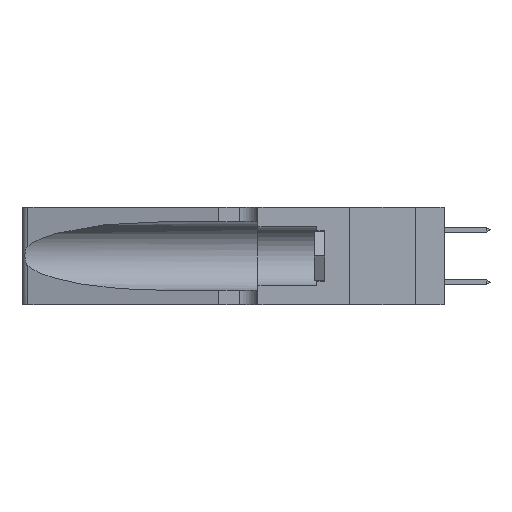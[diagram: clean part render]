
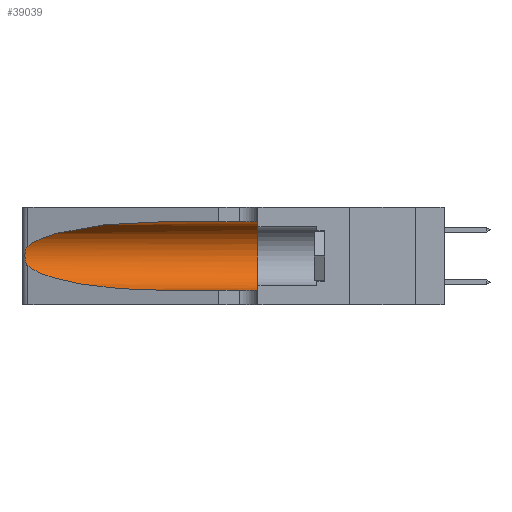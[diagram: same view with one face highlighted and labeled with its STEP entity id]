
A CAD part, left-side view. The second image highlights one B-rep face of the part: STEP entity #39039.
In plain terms, the highlighted cylindrical face has radius 3.308 mm (diameter 6.617 mm), a partial arc.
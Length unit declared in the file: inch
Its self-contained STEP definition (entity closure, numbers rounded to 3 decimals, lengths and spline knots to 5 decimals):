
#1113 = EDGE_CURVE ( 'NONE', #6141, #28850, #5608, .T. ) ;
#3563 =( BOUNDED_CURVE ( )  B_SPLINE_CURVE ( 3, ( #38087, #4190, #41437, #21328 ),
 .UNSPECIFIED., .F., .T. ) 
 B_SPLINE_CURVE_WITH_KNOTS ( ( 4, 4 ),
 ( 3.44316, 4.71239 ),
 .UNSPECIFIED. ) 
 CURVE ( )  GEOMETRIC_REPRESENTATION_ITEM ( )  RATIONAL_B_SPLINE_CURVE ( ( 1., 0.87, 0.87, 1. ) ) 
 REPRESENTATION_ITEM ( '' )  );
#4190 = CARTESIAN_POINT ( 'NONE',  ( 0.2373, 1.15595, 0.08982 ) ) ;
#4416 = CARTESIAN_POINT ( 'NONE',  ( 0.25787, 1.23484, 0.2124 ) ) ;
#5608 = CIRCLE ( 'NONE', #32567, 0.13025 ) ;
#6013 = VERTEX_POINT ( 'NONE', #11095 ) ;
#6141 = VERTEX_POINT ( 'NONE', #38516 ) ;
#6276 = CARTESIAN_POINT ( 'NONE',  ( 0.18966, 0.96281, 0.31525 ) ) ;
#7847 = CARTESIAN_POINT ( 'NONE',  ( 0.26018, 1.23835, 0.19895 ) ) ;
#7897 = ORIENTED_EDGE ( 'NONE', *, *, #31077, .T. ) ;
#8219 =( BOUNDED_CURVE ( )  B_SPLINE_CURVE ( 3, ( #43341, #6276, #33467, #13205 ),
 .UNSPECIFIED., .F., .F. ) 
 B_SPLINE_CURVE_WITH_KNOTS ( ( 4, 4 ),
 ( 1.5708, 2.84003 ),
 .UNSPECIFIED. ) 
 CURVE ( )  GEOMETRIC_REPRESENTATION_ITEM ( )  RATIONAL_B_SPLINE_CURVE ( ( 1., 0.87, 0.87, 1. ) ) 
 REPRESENTATION_ITEM ( '' )  );
#10027 = VECTOR ( 'NONE', #10029, 39.37008 ) ;
#10029 = DIRECTION ( 'NONE',  ( 0., -1., 0. ) ) ;
#11014 = CARTESIAN_POINT ( 'NONE',  ( 0.1305, 1.61858, 0.05475 ) ) ;
#11095 = CARTESIAN_POINT ( 'NONE',  ( 0.25487, 1.22718, 0.14631 ) ) ;
#11128 = LINE ( 'NONE', #26980, #10027 ) ;
#11334 = CARTESIAN_POINT ( 'NONE',  ( 0.26075, 1.23896, 0.178 ) ) ;
#11648 = CARTESIAN_POINT ( 'NONE',  ( 0.1305, 1.61858, 0.185 ) ) ;
#13205 = CARTESIAN_POINT ( 'NONE',  ( 0.25487, 1.22718, 0.22369 ) ) ;
#13450 = DIRECTION ( 'NONE',  ( 0., 1., 0. ) ) ;
#14767 = CARTESIAN_POINT ( 'NONE',  ( 0.25856, 1.23593, 0.16098 ) ) ;
#17105 = FACE_OUTER_BOUND ( 'NONE', #19273, .T. ) ;
#17510 = LINE ( 'NONE', #11014, #43232 ) ;
#17701 = ORIENTED_EDGE ( 'NONE', *, *, #42956, .T. ) ;
#18016 = CARTESIAN_POINT ( 'NONE',  ( 0.25555, 1.22994, 0.2215 ) ) ;
#18171 = CARTESIAN_POINT ( 'NONE',  ( 0.25639, 1.23186, 0.15144 ) ) ;
#18468 = ORIENTED_EDGE ( 'NONE', *, *, #22347, .T. ) ;
#19273 = EDGE_LOOP ( 'NONE', ( #7897, #18468, #27460, #17701, #28132, #34676 ) ) ;
#20178 = EDGE_CURVE ( 'NONE', #6013, #26411, #3563, .T. ) ;
#21328 = CARTESIAN_POINT ( 'NONE',  ( 0.1305, 0.72297, 0.05475 ) ) ;
#21550 = CARTESIAN_POINT ( 'NONE',  ( 0.25487, 1.22718, 0.14631 ) ) ;
#22347 = EDGE_CURVE ( 'NONE', #40003, #6013, #24054, .T. ) ;
#23390 = EDGE_CURVE ( 'NONE', #30802, #6141, #11128, .T. ) ;
#24054 = B_SPLINE_CURVE_WITH_KNOTS ( 'NONE', 3,
 ( #41520, #18016, #24819, #4416, #28243, #7847, #31604, #11334, #34982, #14767, #38313, #18171, #41665, #21550 ),
 .UNSPECIFIED., .F., .F.,
 ( 4, 2, 2, 2, 2, 2, 4 ),
 ( 0., 0.00027, 0.00053, 0.00107, 0.0016, 0.00187, 0.00214 ),
 .UNSPECIFIED. ) ;
#24819 = CARTESIAN_POINT ( 'NONE',  ( 0.25639, 1.23184, 0.21858 ) ) ;
#25011 = CYLINDRICAL_SURFACE ( 'NONE', #41672, 0.13025 ) ;
#25281 = DIRECTION ( 'NONE',  ( 0., -1., 0. ) ) ;
#26039 = CARTESIAN_POINT ( 'NONE',  ( 0.25487, 1.22718, 0.22369 ) ) ;
#26411 = VERTEX_POINT ( 'NONE', #37703 ) ;
#26980 = CARTESIAN_POINT ( 'NONE',  ( 0.1305, 1.61858, 0.31525 ) ) ;
#27460 = ORIENTED_EDGE ( 'NONE', *, *, #20178, .T. ) ;
#28132 = ORIENTED_EDGE ( 'NONE', *, *, #1113, .F. ) ;
#28243 = CARTESIAN_POINT ( 'NONE',  ( 0.25854, 1.2359, 0.20912 ) ) ;
#28850 = VERTEX_POINT ( 'NONE', #32146 ) ;
#30802 = VERTEX_POINT ( 'NONE', #35356 ) ;
#31077 = EDGE_CURVE ( 'NONE', #30802, #40003, #8219, .T. ) ;
#31312 = DIRECTION ( 'NONE',  ( 0., -1., 0. ) ) ;
#31604 = CARTESIAN_POINT ( 'NONE',  ( 0.26075, 1.23896, 0.19203 ) ) ;
#32146 = CARTESIAN_POINT ( 'NONE',  ( 0.1305, 0.35, 0.05475 ) ) ;
#32567 = AXIS2_PLACEMENT_3D ( 'NONE', #33692, #13450, #37013 ) ;
#33467 = CARTESIAN_POINT ( 'NONE',  ( 0.2373, 1.15595, 0.28018 ) ) ;
#33692 = CARTESIAN_POINT ( 'NONE',  ( 0.1305, 0.35, 0.185 ) ) ;
#34676 = ORIENTED_EDGE ( 'NONE', *, *, #23390, .F. ) ;
#34982 = CARTESIAN_POINT ( 'NONE',  ( 0.26017, 1.23833, 0.17102 ) ) ;
#35356 = CARTESIAN_POINT ( 'NONE',  ( 0.1305, 0.72297, 0.31525 ) ) ;
#37013 = DIRECTION ( 'NONE',  ( 0., 0., 1. ) ) ;
#37703 = CARTESIAN_POINT ( 'NONE',  ( 0.1305, 0.72297, 0.05475 ) ) ;
#38087 = CARTESIAN_POINT ( 'NONE',  ( 0.25487, 1.22718, 0.14631 ) ) ;
#38313 = CARTESIAN_POINT ( 'NONE',  ( 0.25789, 1.23486, 0.15765 ) ) ;
#38516 = CARTESIAN_POINT ( 'NONE',  ( 0.1305, 0.35, 0.31525 ) ) ;
#38632 = DIRECTION ( 'NONE',  ( 0., 0., -1. ) ) ;
#39039 = ADVANCED_FACE ( 'NONE', ( #17105 ), #25011, .F. ) ;
#40003 = VERTEX_POINT ( 'NONE', #26039 ) ;
#41437 = CARTESIAN_POINT ( 'NONE',  ( 0.18966, 0.96281, 0.05475 ) ) ;
#41520 = CARTESIAN_POINT ( 'NONE',  ( 0.25487, 1.22718, 0.22369 ) ) ;
#41665 = CARTESIAN_POINT ( 'NONE',  ( 0.25555, 1.22993, 0.14849 ) ) ;
#41672 = AXIS2_PLACEMENT_3D ( 'NONE', #11648, #25281, #38632 ) ;
#42956 = EDGE_CURVE ( 'NONE', #26411, #28850, #17510, .T. ) ;
#43232 = VECTOR ( 'NONE', #31312, 39.37008 ) ;
#43341 = CARTESIAN_POINT ( 'NONE',  ( 0.1305, 0.72297, 0.31525 ) ) ;
